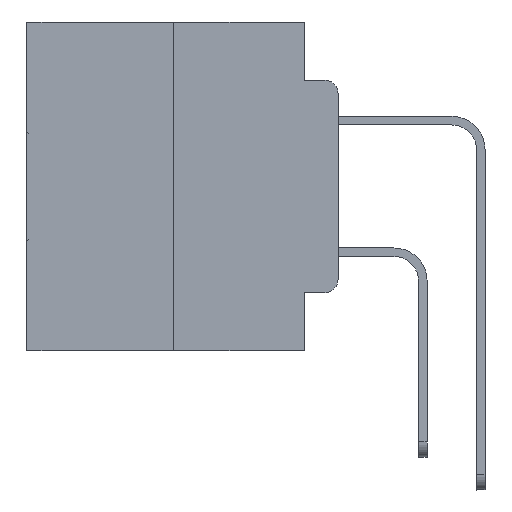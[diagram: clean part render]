
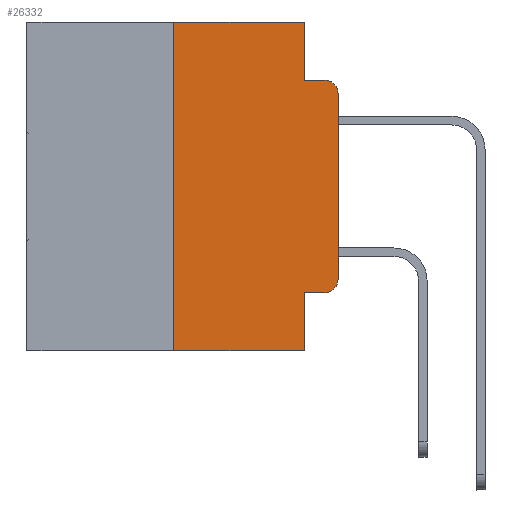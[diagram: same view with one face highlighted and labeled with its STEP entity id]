
A CAD part, left-side view. The second image highlights one B-rep face of the part: STEP entity #26332.
In plain terms, the highlighted planar face has unit normal (-1, 0, 0).
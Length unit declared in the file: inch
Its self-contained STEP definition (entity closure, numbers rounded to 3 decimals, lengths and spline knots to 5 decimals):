
#135 = VERTEX_POINT ( 'NONE', #30906 ) ;
#390 = CARTESIAN_POINT ( 'NONE',  ( 0., 0.473, 0. ) ) ;
#410 = VERTEX_POINT ( 'NONE', #10264 ) ;
#726 = EDGE_CURVE ( 'NONE', #31042, #19181, #31998, .T. ) ;
#1260 = AXIS2_PLACEMENT_3D ( 'NONE', #31558, #21254, #11742 ) ;
#1520 = DIRECTION ( 'NONE',  ( 0., 0., 1. ) ) ;
#2432 = DIRECTION ( 'NONE',  ( 1., 0., 0. ) ) ;
#2758 = CARTESIAN_POINT ( 'NONE',  ( 0., 0.473, 0. ) ) ;
#2857 = LINE ( 'NONE', #390, #23903 ) ;
#3732 = ORIENTED_EDGE ( 'NONE', *, *, #30761, .F. ) ;
#3936 = ORIENTED_EDGE ( 'NONE', *, *, #8492, .T. ) ;
#4439 = EDGE_CURVE ( 'NONE', #27996, #6987, #2857, .T. ) ;
#4481 = EDGE_CURVE ( 'NONE', #24798, #11887, #22482, .T. ) ;
#5304 = DIRECTION ( 'NONE',  ( 0., -1., 0. ) ) ;
#5329 = DIRECTION ( 'NONE',  ( 0., -1., 0. ) ) ;
#5406 = VECTOR ( 'NONE', #8961, 39.37008 ) ;
#5922 = ORIENTED_EDGE ( 'NONE', *, *, #4481, .T. ) ;
#6245 = AXIS2_PLACEMENT_3D ( 'NONE', #2758, #2432, #32056 ) ;
#6616 = ORIENTED_EDGE ( 'NONE', *, *, #12116, .F. ) ;
#6887 = CARTESIAN_POINT ( 'NONE',  ( 0., 0.02, -0.4115 ) ) ;
#6987 = VERTEX_POINT ( 'NONE', #15830 ) ;
#7286 = CIRCLE ( 'NONE', #27151, 0.02 ) ;
#8040 = VECTOR ( 'NONE', #23293, 39.37008 ) ;
#8421 = EDGE_CURVE ( 'NONE', #21208, #19181, #28757, .T. ) ;
#8492 = EDGE_CURVE ( 'NONE', #11887, #410, #27349, .T. ) ;
#8961 = DIRECTION ( 'NONE',  ( 0., 0., -1. ) ) ;
#9258 = LINE ( 'NONE', #14308, #28241 ) ;
#9627 = ORIENTED_EDGE ( 'NONE', *, *, #726, .T. ) ;
#10264 = CARTESIAN_POINT ( 'NONE',  ( 0., 0.02, -0.0885 ) ) ;
#11619 = EDGE_LOOP ( 'NONE', ( #5922, #3936, #6616, #25736, #13281, #3732, #9627, #25535, #18550, #27965 ) ) ;
#11742 = DIRECTION ( 'NONE',  ( 0., 0., -1. ) ) ;
#11887 = VERTEX_POINT ( 'NONE', #21689 ) ;
#12116 = EDGE_CURVE ( 'NONE', #135, #410, #13284, .T. ) ;
#12835 = LINE ( 'NONE', #30181, #18836 ) ;
#13281 = ORIENTED_EDGE ( 'NONE', *, *, #4439, .F. ) ;
#13284 = LINE ( 'NONE', #20176, #8040 ) ;
#13656 = CARTESIAN_POINT ( 'NONE',  ( 0., 0.051, -0.4115 ) ) ;
#13720 = DIRECTION ( 'NONE',  ( -1., 0., 0. ) ) ;
#14288 = DIRECTION ( 'NONE',  ( 0., -1., 0. ) ) ;
#14308 = CARTESIAN_POINT ( 'NONE',  ( 0., 0.051, 0. ) ) ;
#14677 = CARTESIAN_POINT ( 'NONE',  ( 0., 0.051, -0.5 ) ) ;
#15830 = CARTESIAN_POINT ( 'NONE',  ( 0., 0.051, 0. ) ) ;
#15909 = LINE ( 'NONE', #25741, #19223 ) ;
#16875 = EDGE_CURVE ( 'NONE', #6987, #135, #9258, .T. ) ;
#17826 = VERTEX_POINT ( 'NONE', #6887 ) ;
#18550 = ORIENTED_EDGE ( 'NONE', *, *, #26940, .T. ) ;
#18836 = VECTOR ( 'NONE', #5329, 39.37008 ) ;
#19181 = VERTEX_POINT ( 'NONE', #14677 ) ;
#19223 = VECTOR ( 'NONE', #1520, 39.37008 ) ;
#20176 = CARTESIAN_POINT ( 'NONE',  ( 0., 0.051, -0.0885 ) ) ;
#21208 = VERTEX_POINT ( 'NONE', #13656 ) ;
#21254 = DIRECTION ( 'NONE',  ( -1., 0., 0. ) ) ;
#21311 = VECTOR ( 'NONE', #22977, 39.37008 ) ;
#21689 = CARTESIAN_POINT ( 'NONE',  ( 0., 0., -0.1085 ) ) ;
#21909 = VECTOR ( 'NONE', #14288, 39.37008 ) ;
#22077 = PLANE ( 'NONE',  #6245 ) ;
#22482 = LINE ( 'NONE', #23143, #21311 ) ;
#22977 = DIRECTION ( 'NONE',  ( 0., 0., 1. ) ) ;
#23143 = CARTESIAN_POINT ( 'NONE',  ( 0., 0., 0. ) ) ;
#23293 = DIRECTION ( 'NONE',  ( 0., -1., 0. ) ) ;
#23730 = DIRECTION ( 'NONE',  ( 0., 0., -1. ) ) ;
#23903 = VECTOR ( 'NONE', #5304, 39.37008 ) ;
#24298 = CARTESIAN_POINT ( 'NONE',  ( 0., 0.473, -0.5 ) ) ;
#24467 = DIRECTION ( 'NONE',  ( 0., 0., -1. ) ) ;
#24798 = VERTEX_POINT ( 'NONE', #25982 ) ;
#25535 = ORIENTED_EDGE ( 'NONE', *, *, #8421, .F. ) ;
#25736 = ORIENTED_EDGE ( 'NONE', *, *, #16875, .F. ) ;
#25741 = CARTESIAN_POINT ( 'NONE',  ( 0., 0.25, 0. ) ) ;
#25982 = CARTESIAN_POINT ( 'NONE',  ( 0., 0., -0.3915 ) ) ;
#26159 = CARTESIAN_POINT ( 'NONE',  ( 0., 0.02, -0.3915 ) ) ;
#26274 = EDGE_CURVE ( 'NONE', #17826, #24798, #7286, .T. ) ;
#26332 = ADVANCED_FACE ( 'NONE', ( #26958 ), #22077, .F. ) ;
#26940 = EDGE_CURVE ( 'NONE', #21208, #17826, #12835, .T. ) ;
#26958 = FACE_OUTER_BOUND ( 'NONE', #11619, .T. ) ;
#27151 = AXIS2_PLACEMENT_3D ( 'NONE', #26159, #13720, #23730 ) ;
#27349 = CIRCLE ( 'NONE', #1260, 0.02 ) ;
#27965 = ORIENTED_EDGE ( 'NONE', *, *, #26274, .T. ) ;
#27996 = VERTEX_POINT ( 'NONE', #29949 ) ;
#28241 = VECTOR ( 'NONE', #24467, 39.37008 ) ;
#28757 = LINE ( 'NONE', #31217, #5406 ) ;
#29949 = CARTESIAN_POINT ( 'NONE',  ( 0., 0.25, 0. ) ) ;
#30181 = CARTESIAN_POINT ( 'NONE',  ( 0., 0.051, -0.4115 ) ) ;
#30466 = CARTESIAN_POINT ( 'NONE',  ( 0., 0.25, -0.5 ) ) ;
#30761 = EDGE_CURVE ( 'NONE', #31042, #27996, #15909, .T. ) ;
#30906 = CARTESIAN_POINT ( 'NONE',  ( 0., 0.051, -0.0885 ) ) ;
#31042 = VERTEX_POINT ( 'NONE', #30466 ) ;
#31217 = CARTESIAN_POINT ( 'NONE',  ( 0., 0.051, 0. ) ) ;
#31558 = CARTESIAN_POINT ( 'NONE',  ( 0., 0.02, -0.1085 ) ) ;
#31998 = LINE ( 'NONE', #24298, #21909 ) ;
#32056 = DIRECTION ( 'NONE',  ( 0., 0., -1. ) ) ;
